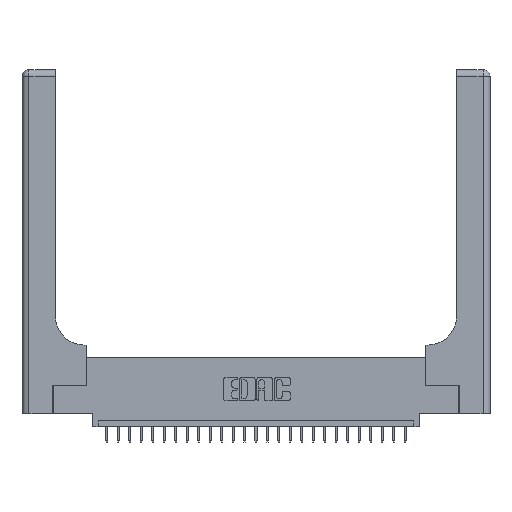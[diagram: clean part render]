
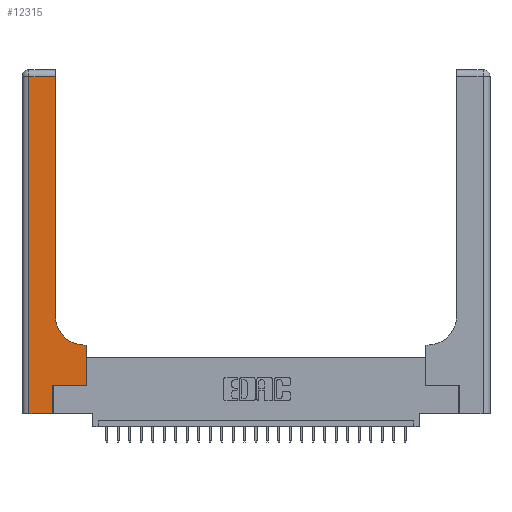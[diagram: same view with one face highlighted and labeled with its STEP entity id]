
A CAD part, top view. The second image highlights one B-rep face of the part: STEP entity #12315.
In plain terms, the highlighted planar face has unit normal (0, 0, 1).
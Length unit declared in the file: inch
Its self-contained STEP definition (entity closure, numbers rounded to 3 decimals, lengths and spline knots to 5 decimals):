
#122 = CARTESIAN_POINT ( 'NONE',  ( 0.2915, 3., 0.37 ) ) ;
#179 = CARTESIAN_POINT ( 'NONE',  ( 0.5585, 0.25, 0.37 ) ) ;
#191 = EDGE_CURVE ( 'NONE', #13214, #20379, #23894, .T. ) ;
#297 = ORIENTED_EDGE ( 'NONE', *, *, #11772, .T. ) ;
#341 = VECTOR ( 'NONE', #1090, 39.37008 ) ;
#1075 = DIRECTION ( 'NONE',  ( 0., 1., 0. ) ) ;
#1090 = DIRECTION ( 'NONE',  ( 1., 0., 0. ) ) ;
#1545 = DIRECTION ( 'NONE',  ( 1., 0., 0. ) ) ;
#1885 = CARTESIAN_POINT ( 'NONE',  ( 0.2915, 0.85, 0.37 ) ) ;
#2107 = DIRECTION ( 'NONE',  ( 0., 0., -1. ) ) ;
#2279 = LINE ( 'NONE', #179, #6757 ) ;
#2373 = LINE ( 'NONE', #8731, #4584 ) ;
#2406 = CARTESIAN_POINT ( 'NONE',  ( 0.06, 2.94, 0.37 ) ) ;
#3185 = AXIS2_PLACEMENT_3D ( 'NONE', #21345, #2107, #1545 ) ;
#3737 = LINE ( 'NONE', #14015, #16806 ) ;
#4584 = VECTOR ( 'NONE', #15034, 39.37008 ) ;
#4687 = DIRECTION ( 'NONE',  ( 0., -1., 0. ) ) ;
#4890 = VERTEX_POINT ( 'NONE', #18975 ) ;
#5380 = VECTOR ( 'NONE', #11394, 39.37008 ) ;
#5586 = CARTESIAN_POINT ( 'NONE',  ( 0.2915, 0.6, 0.37 ) ) ;
#5744 = EDGE_CURVE ( 'NONE', #19996, #24362, #25096, .T. ) ;
#6757 = VECTOR ( 'NONE', #10991, 39.37008 ) ;
#6797 = CARTESIAN_POINT ( 'NONE',  ( 0.06, 3., 0.37 ) ) ;
#7333 = VERTEX_POINT ( 'NONE', #1885 ) ;
#7412 = DIRECTION ( 'NONE',  ( 0., 0., -1. ) ) ;
#8425 = LINE ( 'NONE', #122, #20334 ) ;
#8710 = DIRECTION ( 'NONE',  ( 0., 1., 0. ) ) ;
#8731 = CARTESIAN_POINT ( 'NONE',  ( 0.269, 0.25, 0.37 ) ) ;
#9285 = EDGE_CURVE ( 'NONE', #20379, #21310, #18359, .T. ) ;
#9567 = CARTESIAN_POINT ( 'NONE',  ( 0.5585, 0.25, 0.37 ) ) ;
#9953 = FACE_OUTER_BOUND ( 'NONE', #26926, .T. ) ;
#10487 = VERTEX_POINT ( 'NONE', #9567 ) ;
#10991 = DIRECTION ( 'NONE',  ( 0., 1., 0. ) ) ;
#11394 = DIRECTION ( 'NONE',  ( -1., 0., 0. ) ) ;
#11650 = ORIENTED_EDGE ( 'NONE', *, *, #191, .T. ) ;
#11772 = EDGE_CURVE ( 'NONE', #4890, #13214, #26254, .T. ) ;
#11919 = DIRECTION ( 'NONE',  ( -1., 0., 0. ) ) ;
#12315 = ADVANCED_FACE ( 'NONE', ( #9953 ), #22551, .F. ) ;
#12520 = CARTESIAN_POINT ( 'NONE',  ( 0.269, 0., 0.37 ) ) ;
#13214 = VERTEX_POINT ( 'NONE', #2406 ) ;
#13650 = CARTESIAN_POINT ( 'NONE',  ( 0., 2.94, 0.37 ) ) ;
#14015 = CARTESIAN_POINT ( 'NONE',  ( 0.269, 0., 0.37 ) ) ;
#14360 = EDGE_CURVE ( 'NONE', #10487, #19996, #2279, .T. ) ;
#14707 = EDGE_CURVE ( 'NONE', #24362, #7333, #26493, .T. ) ;
#15034 = DIRECTION ( 'NONE',  ( 1., 0., 0. ) ) ;
#15260 = AXIS2_PLACEMENT_3D ( 'NONE', #26646, #7412, #15984 ) ;
#15270 = CARTESIAN_POINT ( 'NONE',  ( 0.269, 0.25, 0.37 ) ) ;
#15984 = DIRECTION ( 'NONE',  ( -1., 0., 0. ) ) ;
#16507 = EDGE_CURVE ( 'NONE', #25141, #10487, #2373, .T. ) ;
#16806 = VECTOR ( 'NONE', #1075, 39.37008 ) ;
#17630 = ORIENTED_EDGE ( 'NONE', *, *, #5744, .T. ) ;
#18109 = VECTOR ( 'NONE', #11919, 39.37008 ) ;
#18359 = LINE ( 'NONE', #27200, #341 ) ;
#18495 = ORIENTED_EDGE ( 'NONE', *, *, #21786, .T. ) ;
#18963 = ORIENTED_EDGE ( 'NONE', *, *, #16507, .T. ) ;
#18975 = CARTESIAN_POINT ( 'NONE',  ( 0.2915, 2.94, 0.37 ) ) ;
#19568 = VECTOR ( 'NONE', #4687, 39.37008 ) ;
#19996 = VERTEX_POINT ( 'NONE', #25264 ) ;
#20334 = VECTOR ( 'NONE', #8710, 39.37008 ) ;
#20379 = VERTEX_POINT ( 'NONE', #27316 ) ;
#21310 = VERTEX_POINT ( 'NONE', #12520 ) ;
#21345 = CARTESIAN_POINT ( 'NONE',  ( 0.5415, 0.85, 0.37 ) ) ;
#21633 = ORIENTED_EDGE ( 'NONE', *, *, #9285, .T. ) ;
#21786 = EDGE_CURVE ( 'NONE', #7333, #4890, #8425, .T. ) ;
#22075 = EDGE_CURVE ( 'NONE', #21310, #25141, #3737, .T. ) ;
#22467 = CARTESIAN_POINT ( 'NONE',  ( 0.5415, 0.6, 0.37 ) ) ;
#22551 = PLANE ( 'NONE',  #15260 ) ;
#23663 = ORIENTED_EDGE ( 'NONE', *, *, #22075, .T. ) ;
#23894 = LINE ( 'NONE', #6797, #19568 ) ;
#24050 = ORIENTED_EDGE ( 'NONE', *, *, #14360, .T. ) ;
#24362 = VERTEX_POINT ( 'NONE', #22467 ) ;
#25096 = LINE ( 'NONE', #5586, #18109 ) ;
#25141 = VERTEX_POINT ( 'NONE', #15270 ) ;
#25264 = CARTESIAN_POINT ( 'NONE',  ( 0.5585, 0.6, 0.37 ) ) ;
#26254 = LINE ( 'NONE', #13650, #5380 ) ;
#26275 = ORIENTED_EDGE ( 'NONE', *, *, #14707, .T. ) ;
#26493 = CIRCLE ( 'NONE', #3185, 0.25 ) ;
#26646 = CARTESIAN_POINT ( 'NONE',  ( 0., 3., 0.37 ) ) ;
#26926 = EDGE_LOOP ( 'NONE', ( #18495, #297, #11650, #21633, #23663, #18963, #24050, #17630, #26275 ) ) ;
#27200 = CARTESIAN_POINT ( 'NONE',  ( 0., 0., 0.37 ) ) ;
#27316 = CARTESIAN_POINT ( 'NONE',  ( 0.06, 0., 0.37 ) ) ;
